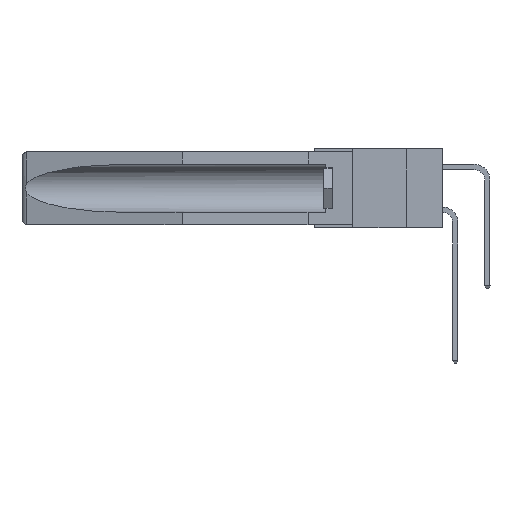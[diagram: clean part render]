
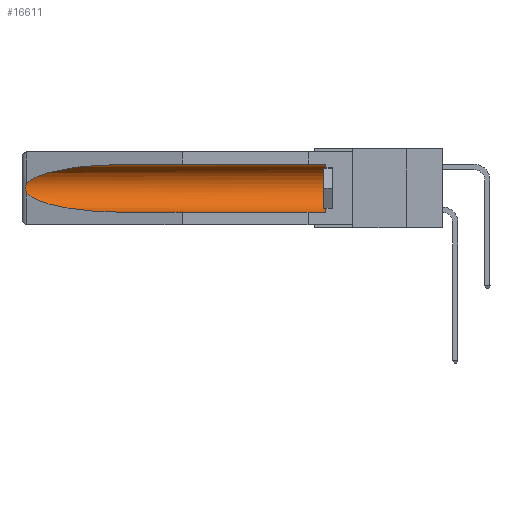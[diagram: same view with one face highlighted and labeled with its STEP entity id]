
A CAD part, left-side view. The second image highlights one B-rep face of the part: STEP entity #16611.
In plain terms, the highlighted cylindrical face has radius 2.857 mm (diameter 5.715 mm), a partial arc.
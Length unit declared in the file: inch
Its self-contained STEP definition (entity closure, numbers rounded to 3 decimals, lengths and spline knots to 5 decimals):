
#88 = ORIENTED_EDGE ( 'NONE', *, *, #27939, .T. ) ;
#891 = CARTESIAN_POINT ( 'NONE',  ( 0.26537, 1.52718, -0.19328 ) ) ;
#2432 = CARTESIAN_POINT ( 'NONE',  ( 0.155, -0.30754, -0.284 ) ) ;
#3779 = VERTEX_POINT ( 'NONE', #30919 ) ;
#4025 = FACE_OUTER_BOUND ( 'NONE', #10637, .T. ) ;
#4532 = ORIENTED_EDGE ( 'NONE', *, *, #18785, .F. ) ;
#6006 = EDGE_CURVE ( 'NONE', #3779, #25713, #6897, .T. ) ;
#6897 = CIRCLE ( 'NONE', #15641, 0.1125 ) ;
#7102 = CARTESIAN_POINT ( 'NONE',  ( 0.21114, 1.30732, -0.059 ) ) ;
#7272 = CARTESIAN_POINT ( 'NONE',  ( 0.26654, 1.53092, -0.15636 ) ) ;
#7425 = CARTESIAN_POINT ( 'NONE',  ( 0.25451, 1.48313, -0.09465 ) ) ;
#7958 = CYLINDRICAL_SURFACE ( 'NONE', #21912, 0.1125 ) ;
#8328 = LINE ( 'NONE', #12158, #15717 ) ;
#9652 = CARTESIAN_POINT ( 'NONE',  ( 0.2673, 1.5327, -0.16383 ) ) ;
#9755 = CARTESIAN_POINT ( 'NONE',  ( 0.26597, 1.5296, -0.19026 ) ) ;
#10046 = ORIENTED_EDGE ( 'NONE', *, *, #24365, .T. ) ;
#10160 = DIRECTION ( 'NONE',  ( 0., 1., 0. ) ) ;
#10481 = CARTESIAN_POINT ( 'NONE',  ( 0.25451, 1.48313, -0.24835 ) ) ;
#10607 = VERTEX_POINT ( 'NONE', #22791 ) ;
#10637 = EDGE_LOOP ( 'NONE', ( #10046, #31541, #88, #4532, #22602, #26083 ) ) ;
#11764 = LINE ( 'NONE', #2432, #19964 ) ;
#12000 = CARTESIAN_POINT ( 'NONE',  ( 0.26537, 1.52718, -0.14972 ) ) ;
#12158 = CARTESIAN_POINT ( 'NONE',  ( 0.155, -0.30754, -0.059 ) ) ;
#12671 = CARTESIAN_POINT ( 'NONE',  ( 0.26537, 1.52718, -0.19328 ) ) ;
#12992 = CARTESIAN_POINT ( 'NONE',  ( 0.21114, 1.30732, -0.284 ) ) ;
#13413 =( BOUNDED_CURVE ( )  B_SPLINE_CURVE ( 3, ( #12671, #10481, #12992, #30181 ),
 .UNSPECIFIED., .F., .T. ) 
 B_SPLINE_CURVE_WITH_KNOTS ( ( 4, 4 ),
 ( 0.1948, 1.5708 ),
 .UNSPECIFIED. ) 
 CURVE ( )  GEOMETRIC_REPRESENTATION_ITEM ( )  RATIONAL_B_SPLINE_CURVE ( ( 1., 0.848, 0.848, 1. ) ) 
 REPRESENTATION_ITEM ( '' )  );
#14030 = CARTESIAN_POINT ( 'NONE',  ( 0.155, 0.126, -0.1715 ) ) ;
#14222 = DIRECTION ( 'NONE',  ( 0., 1., 0. ) ) ;
#15641 = AXIS2_PLACEMENT_3D ( 'NONE', #14030, #21556, #16527 ) ;
#15717 = VECTOR ( 'NONE', #14222, 39.37008 ) ;
#16340 = EDGE_CURVE ( 'NONE', #32252, #19652, #16992, .T. ) ;
#16527 = DIRECTION ( 'NONE',  ( 0., 0., 1. ) ) ;
#16611 = ADVANCED_FACE ( 'NONE', ( #4025 ), #7958, .F. ) ;
#16992 = B_SPLINE_CURVE_WITH_KNOTS ( 'NONE', 3,
 ( #32076, #24606, #7272, #9652, #24713, #27138, #19792, #21849, #9755, #27243 ),
 .UNSPECIFIED., .F., .F.,
 ( 4, 2, 2, 2, 4 ),
 ( 0., 0.00029, 0.00058, 0.00087, 0.00117 ),
 .UNSPECIFIED. ) ;
#17152 = EDGE_CURVE ( 'NONE', #25713, #27994, #8328, .T. ) ;
#18310 = CARTESIAN_POINT ( 'NONE',  ( 0.26537, 1.52718, -0.14972 ) ) ;
#18785 = EDGE_CURVE ( 'NONE', #3779, #10607, #11764, .T. ) ;
#19188 =( BOUNDED_CURVE ( )  B_SPLINE_CURVE ( 3, ( #22372, #7102, #7425, #12000 ),
 .UNSPECIFIED., .F., .F. ) 
 B_SPLINE_CURVE_WITH_KNOTS ( ( 4, 4 ),
 ( 4.71239, 6.08839 ),
 .UNSPECIFIED. ) 
 CURVE ( )  GEOMETRIC_REPRESENTATION_ITEM ( )  RATIONAL_B_SPLINE_CURVE ( ( 1., 0.848, 0.848, 1. ) ) 
 REPRESENTATION_ITEM ( '' )  );
#19652 = VERTEX_POINT ( 'NONE', #891 ) ;
#19792 = CARTESIAN_POINT ( 'NONE',  ( 0.2673, 1.53269, -0.17917 ) ) ;
#19964 = VECTOR ( 'NONE', #10160, 39.37008 ) ;
#20509 = CARTESIAN_POINT ( 'NONE',  ( 0.155, 1.07973, -0.059 ) ) ;
#21556 = DIRECTION ( 'NONE',  ( 0., -1., 0. ) ) ;
#21849 = CARTESIAN_POINT ( 'NONE',  ( 0.26655, 1.53094, -0.18657 ) ) ;
#21912 = AXIS2_PLACEMENT_3D ( 'NONE', #29373, #31899, #26512 ) ;
#22372 = CARTESIAN_POINT ( 'NONE',  ( 0.155, 1.07973, -0.059 ) ) ;
#22602 = ORIENTED_EDGE ( 'NONE', *, *, #6006, .T. ) ;
#22791 = CARTESIAN_POINT ( 'NONE',  ( 0.155, 1.07973, -0.284 ) ) ;
#24365 = EDGE_CURVE ( 'NONE', #27994, #32252, #19188, .T. ) ;
#24606 = CARTESIAN_POINT ( 'NONE',  ( 0.26597, 1.52961, -0.15275 ) ) ;
#24713 = CARTESIAN_POINT ( 'NONE',  ( 0.2675, 1.53308, -0.16763 ) ) ;
#25713 = VERTEX_POINT ( 'NONE', #26397 ) ;
#26083 = ORIENTED_EDGE ( 'NONE', *, *, #17152, .T. ) ;
#26397 = CARTESIAN_POINT ( 'NONE',  ( 0.155, 0.126, -0.059 ) ) ;
#26512 = DIRECTION ( 'NONE',  ( 0., 0., 1. ) ) ;
#27138 = CARTESIAN_POINT ( 'NONE',  ( 0.2675, 1.53308, -0.17534 ) ) ;
#27243 = CARTESIAN_POINT ( 'NONE',  ( 0.26537, 1.52718, -0.19328 ) ) ;
#27939 = EDGE_CURVE ( 'NONE', #19652, #10607, #13413, .T. ) ;
#27994 = VERTEX_POINT ( 'NONE', #20509 ) ;
#29373 = CARTESIAN_POINT ( 'NONE',  ( 0.155, -0.30754, -0.1715 ) ) ;
#30181 = CARTESIAN_POINT ( 'NONE',  ( 0.155, 1.07973, -0.284 ) ) ;
#30919 = CARTESIAN_POINT ( 'NONE',  ( 0.155, 0.126, -0.284 ) ) ;
#31541 = ORIENTED_EDGE ( 'NONE', *, *, #16340, .T. ) ;
#31899 = DIRECTION ( 'NONE',  ( 0., 1., 0. ) ) ;
#32076 = CARTESIAN_POINT ( 'NONE',  ( 0.26537, 1.52718, -0.14972 ) ) ;
#32252 = VERTEX_POINT ( 'NONE', #18310 ) ;
